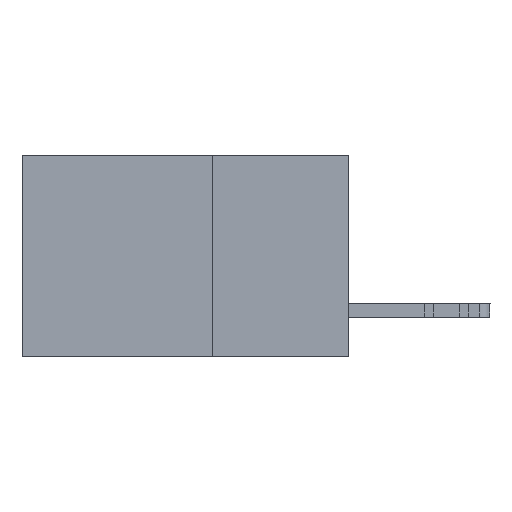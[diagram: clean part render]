
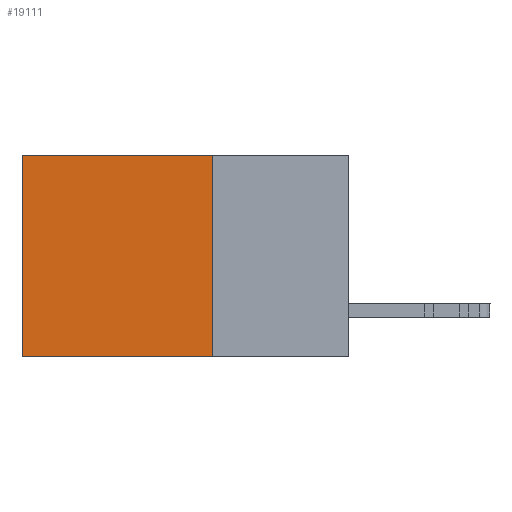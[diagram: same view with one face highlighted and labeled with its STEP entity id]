
A CAD part, left-side view. The second image highlights one B-rep face of the part: STEP entity #19111.
In plain terms, the highlighted planar face has unit normal (-1, 0, 0).
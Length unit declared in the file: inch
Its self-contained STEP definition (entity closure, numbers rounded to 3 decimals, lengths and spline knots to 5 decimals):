
#121 = CARTESIAN_POINT ( 'NONE',  ( 0.2615, 0.6, 0. ) ) ;
#169 = EDGE_CURVE ( 'NONE', #20499, #3933, #17912, .T. ) ;
#1994 = EDGE_CURVE ( 'NONE', #16350, #3933, #4842, .T. ) ;
#2358 = EDGE_CURVE ( 'NONE', #12958, #16350, #10226, .T. ) ;
#2412 = ORIENTED_EDGE ( 'NONE', *, *, #2358, .T. ) ;
#2493 = CARTESIAN_POINT ( 'NONE',  ( 0.2615, 0.25, -0.37 ) ) ;
#3933 = VERTEX_POINT ( 'NONE', #14336 ) ;
#4842 = LINE ( 'NONE', #20317, #23459 ) ;
#5633 = ORIENTED_EDGE ( 'NONE', *, *, #169, .F. ) ;
#6767 = VECTOR ( 'NONE', #10103, 39.37008 ) ;
#7913 = CARTESIAN_POINT ( 'NONE',  ( 0.2615, 0.25, -0.37 ) ) ;
#8902 = CARTESIAN_POINT ( 'NONE',  ( 0.2615, 0.25, 0. ) ) ;
#9849 = DIRECTION ( 'NONE',  ( 0., 0., -1. ) ) ;
#10103 = DIRECTION ( 'NONE',  ( 0., 0., -1. ) ) ;
#10226 = LINE ( 'NONE', #23646, #24863 ) ;
#10734 = EDGE_LOOP ( 'NONE', ( #11164, #5633, #22692, #2412 ) ) ;
#11070 = EDGE_CURVE ( 'NONE', #12958, #20499, #12483, .T. ) ;
#11164 = ORIENTED_EDGE ( 'NONE', *, *, #1994, .T. ) ;
#12483 = LINE ( 'NONE', #13864, #6767 ) ;
#12958 = VERTEX_POINT ( 'NONE', #8902 ) ;
#13864 = CARTESIAN_POINT ( 'NONE',  ( 0.2615, 0.25, -0.37 ) ) ;
#14336 = CARTESIAN_POINT ( 'NONE',  ( 0.2615, 0.6, -0.37 ) ) ;
#14680 = AXIS2_PLACEMENT_3D ( 'NONE', #7913, #21360, #9849 ) ;
#16350 = VERTEX_POINT ( 'NONE', #121 ) ;
#17912 = LINE ( 'NONE', #20290, #22379 ) ;
#19111 = ADVANCED_FACE ( 'NONE', ( #24770 ), #19451, .F. ) ;
#19451 = PLANE ( 'NONE',  #14680 ) ;
#20290 = CARTESIAN_POINT ( 'NONE',  ( 0.2615, 0.25, -0.37 ) ) ;
#20317 = CARTESIAN_POINT ( 'NONE',  ( 0.2615, 0.6, -0.37 ) ) ;
#20449 = DIRECTION ( 'NONE',  ( 0., 1., 0. ) ) ;
#20499 = VERTEX_POINT ( 'NONE', #2493 ) ;
#20765 = DIRECTION ( 'NONE',  ( 0., 0., -1. ) ) ;
#21360 = DIRECTION ( 'NONE',  ( 1., 0., 0. ) ) ;
#22379 = VECTOR ( 'NONE', #20449, 39.37008 ) ;
#22692 = ORIENTED_EDGE ( 'NONE', *, *, #11070, .F. ) ;
#23459 = VECTOR ( 'NONE', #20765, 39.37008 ) ;
#23520 = DIRECTION ( 'NONE',  ( 0., 1., 0. ) ) ;
#23646 = CARTESIAN_POINT ( 'NONE',  ( 0.2615, 0.25, 0. ) ) ;
#24770 = FACE_OUTER_BOUND ( 'NONE', #10734, .T. ) ;
#24863 = VECTOR ( 'NONE', #23520, 39.37008 ) ;
